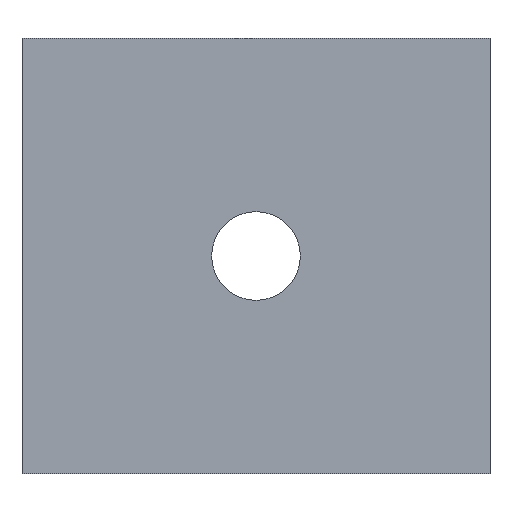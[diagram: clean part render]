
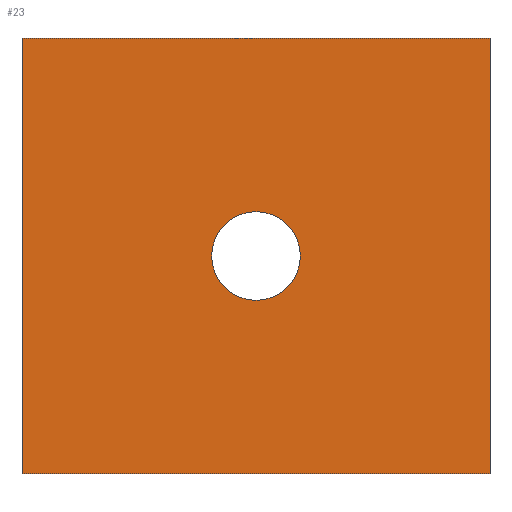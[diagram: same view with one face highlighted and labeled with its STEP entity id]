
A CAD part, front view. The second image highlights one B-rep face of the part: STEP entity #23.
In plain terms, the highlighted planar face has unit normal (0, -1, 0).
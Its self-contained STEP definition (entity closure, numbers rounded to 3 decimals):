
#18 = AXIS2_PLACEMENT_3D ( 'NONE', #113, #408, #154 ) ;
#23 = ADVANCED_FACE ( 'NONE', ( #257, #264 ), #378, .T. ) ;
#26 = EDGE_CURVE ( 'NONE', #211, #427, #458, .T. ) ;
#35 = CARTESIAN_POINT ( 'NONE',  ( 14.5, 0., 13.5 ) ) ;
#39 = VECTOR ( 'NONE', #417, 1000. ) ;
#46 = AXIS2_PLACEMENT_3D ( 'NONE', #122, #415, #163 ) ;
#49 = CIRCLE ( 'NONE', #46, 2.75 ) ;
#87 = VERTEX_POINT ( 'NONE', #35 ) ;
#106 = CARTESIAN_POINT ( 'NONE',  ( -14.5, 0., 13.5 ) ) ;
#113 = CARTESIAN_POINT ( 'NONE',  ( 0., 0., 0. ) ) ;
#115 = LINE ( 'NONE', #171, #317 ) ;
#117 = AXIS2_PLACEMENT_3D ( 'NONE', #412, #373, #369 ) ;
#122 = CARTESIAN_POINT ( 'NONE',  ( 0., 0., 0. ) ) ;
#123 = CARTESIAN_POINT ( 'NONE',  ( -14.5, 0., 13.5 ) ) ;
#128 = CIRCLE ( 'NONE', #18, 2.75 ) ;
#133 = VECTOR ( 'NONE', #326, 1000. ) ;
#143 = EDGE_LOOP ( 'NONE', ( #238, #363, #381, #490 ) ) ;
#146 = CARTESIAN_POINT ( 'NONE',  ( 14.5, 0., -13.5 ) ) ;
#154 = DIRECTION ( 'NONE',  ( 0., 0., 1. ) ) ;
#163 = DIRECTION ( 'NONE',  ( 0., 0., 1. ) ) ;
#171 = CARTESIAN_POINT ( 'NONE',  ( 14.5, 0., 13.5 ) ) ;
#179 = LINE ( 'NONE', #106, #250 ) ;
#182 = ORIENTED_EDGE ( 'NONE', *, *, #397, .T. ) ;
#211 = VERTEX_POINT ( 'NONE', #146 ) ;
#217 = EDGE_CURVE ( 'NONE', #427, #438, #179, .T. ) ;
#238 = ORIENTED_EDGE ( 'NONE', *, *, #473, .F. ) ;
#246 = CARTESIAN_POINT ( 'NONE',  ( 0., 0., -2.75 ) ) ;
#249 = CARTESIAN_POINT ( 'NONE',  ( 0., 0., 2.75 ) ) ;
#250 = VECTOR ( 'NONE', #267, 1000. ) ;
#252 = LINE ( 'NONE', #123, #39 ) ;
#257 = FACE_OUTER_BOUND ( 'NONE', #143, .T. ) ;
#264 = FACE_BOUND ( 'NONE', #472, .T. ) ;
#267 = DIRECTION ( 'NONE',  ( 0., 0., 1. ) ) ;
#292 = DIRECTION ( 'NONE',  ( 0., 0., -1. ) ) ;
#293 = EDGE_CURVE ( 'NONE', #429, #443, #128, .T. ) ;
#317 = VECTOR ( 'NONE', #292, 1000. ) ;
#326 = DIRECTION ( 'NONE',  ( -1., 0., 0. ) ) ;
#329 = CARTESIAN_POINT ( 'NONE',  ( -14.5, 0., -13.5 ) ) ;
#330 = CARTESIAN_POINT ( 'NONE',  ( -14.5, 0., 13.5 ) ) ;
#363 = ORIENTED_EDGE ( 'NONE', *, *, #409, .F. ) ;
#369 = DIRECTION ( 'NONE',  ( 0., 0., -1. ) ) ;
#373 = DIRECTION ( 'NONE',  ( 0., -1., 0. ) ) ;
#378 = PLANE ( 'NONE',  #117 ) ;
#381 = ORIENTED_EDGE ( 'NONE', *, *, #217, .F. ) ;
#391 = ORIENTED_EDGE ( 'NONE', *, *, #293, .T. ) ;
#397 = EDGE_CURVE ( 'NONE', #443, #429, #49, .T. ) ;
#408 = DIRECTION ( 'NONE',  ( 0., 1., 0. ) ) ;
#409 = EDGE_CURVE ( 'NONE', #438, #87, #252, .T. ) ;
#412 = CARTESIAN_POINT ( 'NONE',  ( 0., 0., 0. ) ) ;
#415 = DIRECTION ( 'NONE',  ( 0., 1., 0. ) ) ;
#417 = DIRECTION ( 'NONE',  ( 1., 0., 0. ) ) ;
#427 = VERTEX_POINT ( 'NONE', #499 ) ;
#429 = VERTEX_POINT ( 'NONE', #246 ) ;
#438 = VERTEX_POINT ( 'NONE', #330 ) ;
#443 = VERTEX_POINT ( 'NONE', #249 ) ;
#458 = LINE ( 'NONE', #329, #133 ) ;
#472 = EDGE_LOOP ( 'NONE', ( #391, #182 ) ) ;
#473 = EDGE_CURVE ( 'NONE', #87, #211, #115, .T. ) ;
#490 = ORIENTED_EDGE ( 'NONE', *, *, #26, .F. ) ;
#499 = CARTESIAN_POINT ( 'NONE',  ( -14.5, 0., -13.5 ) ) ;
